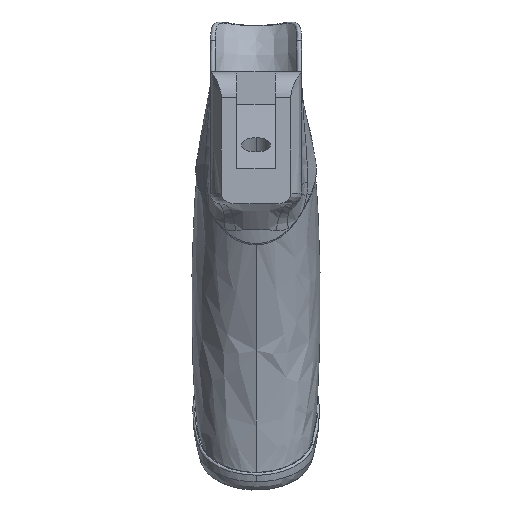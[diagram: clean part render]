
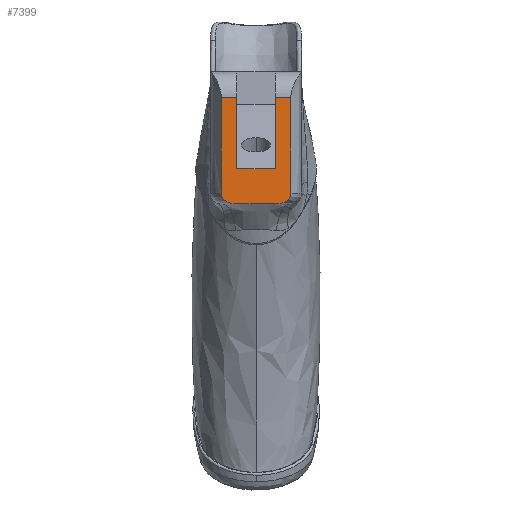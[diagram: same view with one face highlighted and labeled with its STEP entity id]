
A CAD part, top view. The second image highlights one B-rep face of the part: STEP entity #7399.
In plain terms, the highlighted planar face has unit normal (0, 0, 1).
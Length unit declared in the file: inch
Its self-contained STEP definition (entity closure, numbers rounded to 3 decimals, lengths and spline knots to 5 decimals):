
#15 = CARTESIAN_POINT ( 'NONE',  ( 0.187, -0.25, 0. ) ) ;
#17 = CARTESIAN_POINT ( 'NONE',  ( 0.25938, -1.27077, 0. ) ) ;
#143 = CARTESIAN_POINT ( 'NONE',  ( 0.33197, -1.20871, 0. ) ) ;
#314 = VERTEX_POINT ( 'NONE', #15433 ) ;
#655 = DIRECTION ( 'NONE',  ( 0., -1., 0. ) ) ;
#1015 = CARTESIAN_POINT ( 'NONE',  ( -0.32875, -1.21558, 0. ) ) ;
#1138 = LINE ( 'NONE', #20386, #13782 ) ;
#1140 = LINE ( 'NONE', #7195, #22201 ) ;
#1242 = EDGE_CURVE ( 'NONE', #12760, #22358, #11048, .T. ) ;
#1347 = DIRECTION ( 'NONE',  ( 1., 0., 0. ) ) ;
#1394 = B_SPLINE_CURVE_WITH_KNOTS ( 'NONE', 3,
 ( #8457, #24298, #2886, #10594, #1015, #20257, #18229, #16347, #24059, #14467, #22155, #10970, #21013, #18975, #9074, #19107 ),
 .UNSPECIFIED., .F., .F.,
 ( 4, 2, 2, 2, 2, 2, 2, 4 ),
 ( 0., 0.00058, 0.00115, 0.00173, 0.0023, 0.00345, 0.00403, 0.0046 ),
 .UNSPECIFIED. ) ;
#2124 = CARTESIAN_POINT ( 'NONE',  ( -0.2069, -1.2789, 0. ) ) ;
#2874 = LINE ( 'NONE', #10836, #23847 ) ;
#2886 = CARTESIAN_POINT ( 'NONE',  ( -0.33636, -1.19404, 0. ) ) ;
#3387 = DIRECTION ( 'NONE',  ( 0., -1., 0. ) ) ;
#3917 = CARTESIAN_POINT ( 'NONE',  ( 0.30534, -1.24507, 0. ) ) ;
#4842 = ORIENTED_EDGE ( 'NONE', *, *, #11303, .F. ) ;
#5334 = ORIENTED_EDGE ( 'NONE', *, *, #13460, .F. ) ;
#5503 = LINE ( 'NONE', #14934, #16950 ) ;
#5800 = CARTESIAN_POINT ( 'NONE',  ( 0.29941, -1.24989, 0. ) ) ;
#6819 = DIRECTION ( 'NONE',  ( 1., 0., 0. ) ) ;
#6970 = VECTOR ( 'NONE', #655, 39.37008 ) ;
#7002 = VERTEX_POINT ( 'NONE', #22679 ) ;
#7195 = CARTESIAN_POINT ( 'NONE',  ( 0.3375, -1.2789, 0. ) ) ;
#7386 = DIRECTION ( 'NONE',  ( 1., 0., 0. ) ) ;
#7399 = ADVANCED_FACE ( 'NONE', ( #14683 ), #13047, .T. ) ;
#7698 = CARTESIAN_POINT ( 'NONE',  ( 0.26655, -1.26818, 0. ) ) ;
#7765 = CARTESIAN_POINT ( 'NONE',  ( -0.4425, -0.25, 0. ) ) ;
#7825 = CARTESIAN_POINT ( 'NONE',  ( 0.33636, -1.19408, 0. ) ) ;
#8457 = CARTESIAN_POINT ( 'NONE',  ( -0.3375, -1.1789, 0. ) ) ;
#8907 = CARTESIAN_POINT ( 'NONE',  ( 0.3375, -1.1789, 0. ) ) ;
#9074 = CARTESIAN_POINT ( 'NONE',  ( -0.21452, -1.2789, 0. ) ) ;
#9346 = VECTOR ( 'NONE', #1347, 39.37008 ) ;
#9590 = CARTESIAN_POINT ( 'NONE',  ( 0.22262, -1.2789, 0. ) ) ;
#9720 = CARTESIAN_POINT ( 'NONE',  ( 0.3208, -1.22844, 0. ) ) ;
#10445 = CARTESIAN_POINT ( 'NONE',  ( 0.187, -0.94, 0. ) ) ;
#10549 = AXIS2_PLACEMENT_3D ( 'NONE', #16556, #12918, #11060 ) ;
#10594 = CARTESIAN_POINT ( 'NONE',  ( -0.33199, -1.20859, 0. ) ) ;
#10805 = VERTEX_POINT ( 'NONE', #15130 ) ;
#10836 = CARTESIAN_POINT ( 'NONE',  ( 0.187, 0., 0. ) ) ;
#10970 = CARTESIAN_POINT ( 'NONE',  ( -0.24455, -1.27484, 0. ) ) ;
#11048 = LINE ( 'NONE', #16422, #15350 ) ;
#11060 = DIRECTION ( 'NONE',  ( 0., -1., 0. ) ) ;
#11303 = EDGE_CURVE ( 'NONE', #7002, #314, #5503, .T. ) ;
#11591 = CARTESIAN_POINT ( 'NONE',  ( 0.31598, -1.2344, 0. ) ) ;
#12172 = EDGE_CURVE ( 'NONE', #314, #10805, #22372, .T. ) ;
#12544 = VECTOR ( 'NONE', #22408, 39.37008 ) ;
#12752 = VERTEX_POINT ( 'NONE', #15 ) ;
#12760 = VERTEX_POINT ( 'NONE', #2124 ) ;
#12918 = DIRECTION ( 'NONE',  ( 0., 0., 1. ) ) ;
#13047 = PLANE ( 'NONE',  #10549 ) ;
#13460 = EDGE_CURVE ( 'NONE', #12752, #13889, #14473, .T. ) ;
#13590 = EDGE_CURVE ( 'NONE', #21617, #13889, #1140, .T. ) ;
#13782 = VECTOR ( 'NONE', #6819, 39.37008 ) ;
#13885 = EDGE_CURVE ( 'NONE', #22358, #21617, #20167, .T. ) ;
#13889 = VERTEX_POINT ( 'NONE', #17843 ) ;
#14127 = VERTEX_POINT ( 'NONE', #10445 ) ;
#14421 = ORIENTED_EDGE ( 'NONE', *, *, #13885, .T. ) ;
#14450 = EDGE_LOOP ( 'NONE', ( #24011, #14421, #20839, #5334, #14916, #24498, #22840, #17058, #4842, #24850 ) ) ;
#14467 = CARTESIAN_POINT ( 'NONE',  ( -0.28033, -1.26259, 0. ) ) ;
#14473 = LINE ( 'NONE', #22161, #12544 ) ;
#14683 = FACE_OUTER_BOUND ( 'NONE', #14450, .T. ) ;
#14916 = ORIENTED_EDGE ( 'NONE', *, *, #20951, .T. ) ;
#14934 = CARTESIAN_POINT ( 'NONE',  ( -0.3375, -1.2789, 0. ) ) ;
#15130 = CARTESIAN_POINT ( 'NONE',  ( -0.188, -0.25, 0. ) ) ;
#15346 = CARTESIAN_POINT ( 'NONE',  ( 0.28026, -1.26198, 0. ) ) ;
#15350 = VECTOR ( 'NONE', #7386, 39.37008 ) ;
#15433 = CARTESIAN_POINT ( 'NONE',  ( -0.3375, -0.25, 0. ) ) ;
#15474 = CARTESIAN_POINT ( 'NONE',  ( 0.3375, -1.18656, 0. ) ) ;
#16347 = CARTESIAN_POINT ( 'NONE',  ( -0.30517, -1.2451, 0. ) ) ;
#16422 = CARTESIAN_POINT ( 'NONE',  ( -0.4425, -1.2789, 0. ) ) ;
#16556 = CARTESIAN_POINT ( 'NONE',  ( -0.4425, -0.25, 0. ) ) ;
#16722 = DIRECTION ( 'NONE',  ( 0., 1., 0. ) ) ;
#16914 = EDGE_CURVE ( 'NONE', #10805, #18710, #21790, .T. ) ;
#16950 = VECTOR ( 'NONE', #20609, 39.37008 ) ;
#17058 = ORIENTED_EDGE ( 'NONE', *, *, #12172, .F. ) ;
#17068 = EDGE_CURVE ( 'NONE', #18710, #14127, #1138, .T. ) ;
#17231 = CARTESIAN_POINT ( 'NONE',  ( 0.23752, -1.27691, 0. ) ) ;
#17358 = CARTESIAN_POINT ( 'NONE',  ( 0.3288, -1.21555, 0. ) ) ;
#17843 = CARTESIAN_POINT ( 'NONE',  ( 0.3375, -0.25, 0. ) ) ;
#17874 = CARTESIAN_POINT ( 'NONE',  ( -0.188, 0., 0. ) ) ;
#18229 = CARTESIAN_POINT ( 'NONE',  ( -0.31587, -1.23443, 0. ) ) ;
#18710 = VERTEX_POINT ( 'NONE', #22087 ) ;
#18975 = CARTESIAN_POINT ( 'NONE',  ( -0.22208, -1.27839, 0. ) ) ;
#19107 = CARTESIAN_POINT ( 'NONE',  ( -0.2069, -1.2789, 0. ) ) ;
#19497 = CARTESIAN_POINT ( 'NONE',  ( 0.20741, -1.2789, 0. ) ) ;
#20167 = B_SPLINE_CURVE_WITH_KNOTS ( 'NONE', 3,
 ( #21018, #9590, #17231, #17, #7698, #15346, #23049, #5800, #3917, #11591, #9720, #17358, #143, #7825, #15474, #23173 ),
 .UNSPECIFIED., .F., .F.,
 ( 4, 2, 2, 2, 2, 2, 2, 4 ),
 ( 0., 0.00115, 0.00172, 0.00229, 0.00286, 0.00344, 0.00401, 0.00458 ),
 .UNSPECIFIED. ) ;
#20257 = CARTESIAN_POINT ( 'NONE',  ( -0.32073, -1.22843, 0. ) ) ;
#20386 = CARTESIAN_POINT ( 'NONE',  ( -0.188, -0.94, 0. ) ) ;
#20609 = DIRECTION ( 'NONE',  ( 0., 1., 0. ) ) ;
#20839 = ORIENTED_EDGE ( 'NONE', *, *, #13590, .T. ) ;
#20951 = EDGE_CURVE ( 'NONE', #12752, #14127, #2874, .T. ) ;
#21013 = CARTESIAN_POINT ( 'NONE',  ( -0.23707, -1.27637, 0. ) ) ;
#21018 = CARTESIAN_POINT ( 'NONE',  ( 0.20741, -1.2789, 0. ) ) ;
#21617 = VERTEX_POINT ( 'NONE', #8907 ) ;
#21790 = LINE ( 'NONE', #17874, #6970 ) ;
#22087 = CARTESIAN_POINT ( 'NONE',  ( -0.188, -0.94, 0. ) ) ;
#22155 = CARTESIAN_POINT ( 'NONE',  ( -0.26647, -1.26868, 0. ) ) ;
#22161 = CARTESIAN_POINT ( 'NONE',  ( -0.4425, -0.25, 0. ) ) ;
#22201 = VECTOR ( 'NONE', #16722, 39.37008 ) ;
#22358 = VERTEX_POINT ( 'NONE', #19497 ) ;
#22372 = LINE ( 'NONE', #7765, #9346 ) ;
#22408 = DIRECTION ( 'NONE',  ( 1., 0., 0. ) ) ;
#22679 = CARTESIAN_POINT ( 'NONE',  ( -0.3375, -1.1789, 0. ) ) ;
#22840 = ORIENTED_EDGE ( 'NONE', *, *, #16914, .F. ) ;
#23049 = CARTESIAN_POINT ( 'NONE',  ( 0.28685, -1.25835, 0. ) ) ;
#23173 = CARTESIAN_POINT ( 'NONE',  ( 0.3375, -1.1789, 0. ) ) ;
#23847 = VECTOR ( 'NONE', #3387, 39.37008 ) ;
#24011 = ORIENTED_EDGE ( 'NONE', *, *, #1242, .T. ) ;
#24059 = CARTESIAN_POINT ( 'NONE',  ( -0.29931, -1.24986, 0. ) ) ;
#24165 = EDGE_CURVE ( 'NONE', #7002, #12760, #1394, .T. ) ;
#24298 = CARTESIAN_POINT ( 'NONE',  ( -0.3375, -1.18657, 0. ) ) ;
#24498 = ORIENTED_EDGE ( 'NONE', *, *, #17068, .F. ) ;
#24850 = ORIENTED_EDGE ( 'NONE', *, *, #24165, .T. ) ;
